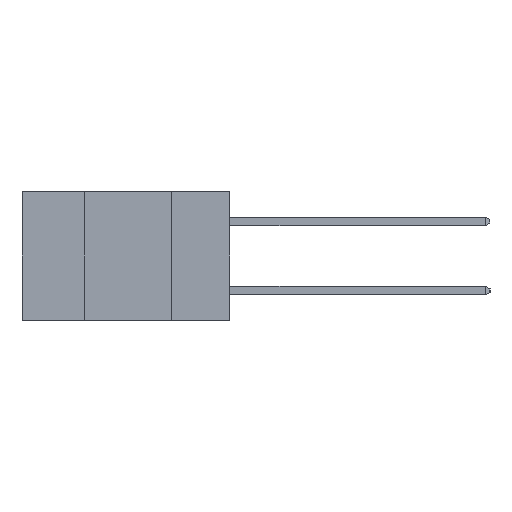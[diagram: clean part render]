
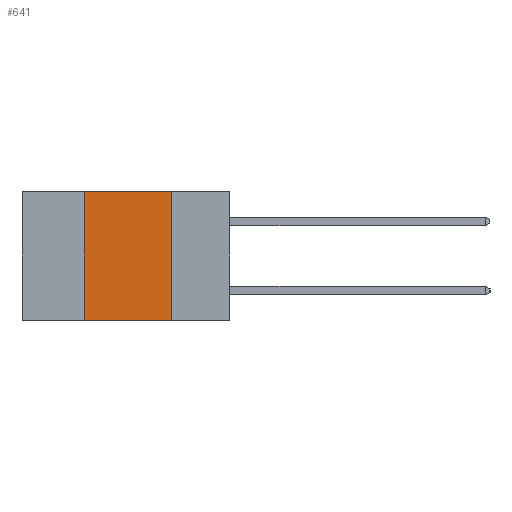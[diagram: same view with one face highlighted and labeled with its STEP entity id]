
A CAD part, left-side view. The second image highlights one B-rep face of the part: STEP entity #641.
In plain terms, the highlighted planar face has unit normal (-1, 0, 0).
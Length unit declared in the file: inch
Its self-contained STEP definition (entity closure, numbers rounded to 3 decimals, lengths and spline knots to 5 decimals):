
#641 = ADVANCED_FACE ( 'NONE', ( #16478 ), #6363, .F. ) ;
#1827 = EDGE_CURVE ( 'NONE', #14914, #5668, #22066, .T. ) ;
#1872 = DIRECTION ( 'NONE',  ( 0., 0., -1. ) ) ;
#3194 = EDGE_CURVE ( 'NONE', #17037, #3395, #7263, .T. ) ;
#3395 = VERTEX_POINT ( 'NONE', #13165 ) ;
#4647 = CARTESIAN_POINT ( 'NONE',  ( 0., 0.17, -0.37 ) ) ;
#4938 = VECTOR ( 'NONE', #11185, 39.37008 ) ;
#5668 = VERTEX_POINT ( 'NONE', #25402 ) ;
#6363 = PLANE ( 'NONE',  #8109 ) ;
#6988 = EDGE_CURVE ( 'NONE', #17037, #14914, #20990, .T. ) ;
#7156 = ORIENTED_EDGE ( 'NONE', *, *, #3194, .T. ) ;
#7263 = LINE ( 'NONE', #18159, #11390 ) ;
#8109 = AXIS2_PLACEMENT_3D ( 'NONE', #11453, #11423, #1872 ) ;
#10438 = LINE ( 'NONE', #4647, #20422 ) ;
#11128 = CARTESIAN_POINT ( 'NONE',  ( 0., 0.42, -0.37 ) ) ;
#11185 = DIRECTION ( 'NONE',  ( 0., 0., 1. ) ) ;
#11390 = VECTOR ( 'NONE', #18045, 39.37008 ) ;
#11423 = DIRECTION ( 'NONE',  ( 1., 0., 0. ) ) ;
#11453 = CARTESIAN_POINT ( 'NONE',  ( 0., 0.6, 0. ) ) ;
#13165 = CARTESIAN_POINT ( 'NONE',  ( 0., 0.17, -0.37 ) ) ;
#14685 = DIRECTION ( 'NONE',  ( 0., 0., -1. ) ) ;
#14914 = VERTEX_POINT ( 'NONE', #18572 ) ;
#15729 = ORIENTED_EDGE ( 'NONE', *, *, #1827, .F. ) ;
#15889 = ORIENTED_EDGE ( 'NONE', *, *, #23906, .F. ) ;
#16478 = FACE_OUTER_BOUND ( 'NONE', #17777, .T. ) ;
#17037 = VERTEX_POINT ( 'NONE', #22751 ) ;
#17777 = EDGE_LOOP ( 'NONE', ( #15889, #15729, #21698, #7156 ) ) ;
#18045 = DIRECTION ( 'NONE',  ( 0., -1., 0. ) ) ;
#18159 = CARTESIAN_POINT ( 'NONE',  ( 0., 0.6, -0.37 ) ) ;
#18572 = CARTESIAN_POINT ( 'NONE',  ( 0., 0.42, 0. ) ) ;
#20422 = VECTOR ( 'NONE', #14685, 39.37008 ) ;
#20990 = LINE ( 'NONE', #11128, #4938 ) ;
#21421 = VECTOR ( 'NONE', #23724, 39.37008 ) ;
#21698 = ORIENTED_EDGE ( 'NONE', *, *, #6988, .F. ) ;
#22066 = LINE ( 'NONE', #24777, #21421 ) ;
#22751 = CARTESIAN_POINT ( 'NONE',  ( 0., 0.42, -0.37 ) ) ;
#23724 = DIRECTION ( 'NONE',  ( 0., -1., 0. ) ) ;
#23906 = EDGE_CURVE ( 'NONE', #5668, #3395, #10438, .T. ) ;
#24777 = CARTESIAN_POINT ( 'NONE',  ( 0., 0.6, 0. ) ) ;
#25402 = CARTESIAN_POINT ( 'NONE',  ( 0., 0.17, 0. ) ) ;
